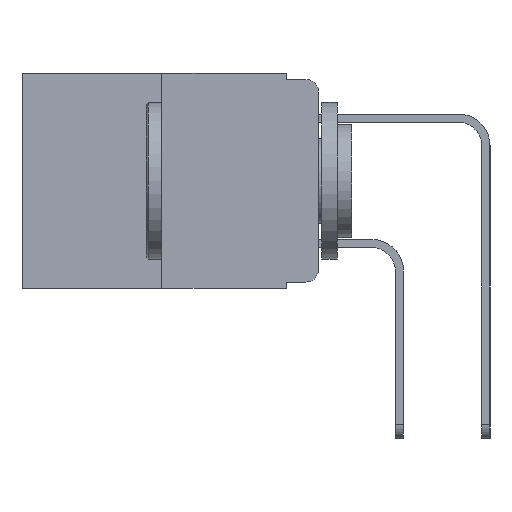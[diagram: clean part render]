
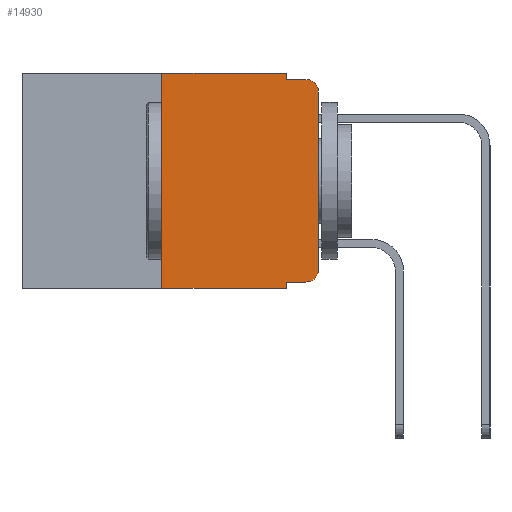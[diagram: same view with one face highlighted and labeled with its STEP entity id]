
A CAD part, left-side view. The second image highlights one B-rep face of the part: STEP entity #14930.
In plain terms, the highlighted planar face has unit normal (-1, 0, 0).
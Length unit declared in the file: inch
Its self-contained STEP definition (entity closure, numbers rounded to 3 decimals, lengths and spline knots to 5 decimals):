
#291 = DIRECTION ( 'NONE',  ( 0., 0., -1. ) ) ;
#442 = VERTEX_POINT ( 'NONE', #15512 ) ;
#761 = ORIENTED_EDGE ( 'NONE', *, *, #16289, .T. ) ;
#1004 = VECTOR ( 'NONE', #14730, 39.37008 ) ;
#1028 = ORIENTED_EDGE ( 'NONE', *, *, #16645, .F. ) ;
#1075 = VERTEX_POINT ( 'NONE', #9823 ) ;
#1347 = CARTESIAN_POINT ( 'NONE',  ( 0., 0.051, -0.01 ) ) ;
#1717 = FACE_OUTER_BOUND ( 'NONE', #5177, .T. ) ;
#1887 = LINE ( 'NONE', #19384, #17419 ) ;
#1895 = VERTEX_POINT ( 'NONE', #10454 ) ;
#1928 = VERTEX_POINT ( 'NONE', #13494 ) ;
#2020 = ORIENTED_EDGE ( 'NONE', *, *, #15933, .T. ) ;
#2046 = DIRECTION ( 'NONE',  ( 1., 0., 0. ) ) ;
#2171 = AXIS2_PLACEMENT_3D ( 'NONE', #11753, #2614, #13213 ) ;
#2304 = ORIENTED_EDGE ( 'NONE', *, *, #16283, .F. ) ;
#2614 = DIRECTION ( 'NONE',  ( -1., 0., 0. ) ) ;
#2619 = ORIENTED_EDGE ( 'NONE', *, *, #8684, .F. ) ;
#2909 = EDGE_CURVE ( 'NONE', #11151, #13283, #9089, .T. ) ;
#3618 = VECTOR ( 'NONE', #8699, 39.37008 ) ;
#3815 = DIRECTION ( 'NONE',  ( -1., 0., 0. ) ) ;
#3822 = CIRCLE ( 'NONE', #2171, 0.02 ) ;
#3830 = ORIENTED_EDGE ( 'NONE', *, *, #4227, .F. ) ;
#4227 = EDGE_CURVE ( 'NONE', #1895, #9646, #1887, .T. ) ;
#4546 = DIRECTION ( 'NONE',  ( 0., 0., 1. ) ) ;
#4596 = EDGE_CURVE ( 'NONE', #1075, #9885, #11877, .T. ) ;
#4952 = DIRECTION ( 'NONE',  ( 0., -1., 0. ) ) ;
#5177 = EDGE_LOOP ( 'NONE', ( #8118, #2020, #2304, #1028, #3830, #2619, #761, #13155, #13760, #7989 ) ) ;
#5407 = CARTESIAN_POINT ( 'NONE',  ( 0., 0.051, -0.343 ) ) ;
#5734 = CARTESIAN_POINT ( 'NONE',  ( 0., 0.051, -0.333 ) ) ;
#7221 = LINE ( 'NONE', #17619, #3618 ) ;
#7349 = CARTESIAN_POINT ( 'NONE',  ( 0., 0.02, -0.01 ) ) ;
#7453 = VERTEX_POINT ( 'NONE', #1347 ) ;
#7605 = DIRECTION ( 'NONE',  ( 0., -1., 0. ) ) ;
#7761 = LINE ( 'NONE', #15059, #15226 ) ;
#7989 = ORIENTED_EDGE ( 'NONE', *, *, #2909, .T. ) ;
#8118 = ORIENTED_EDGE ( 'NONE', *, *, #18871, .T. ) ;
#8357 = VECTOR ( 'NONE', #9488, 39.37008 ) ;
#8454 = CARTESIAN_POINT ( 'NONE',  ( 0., 0.051, 0. ) ) ;
#8684 = EDGE_CURVE ( 'NONE', #1928, #1895, #7761, .T. ) ;
#8699 = DIRECTION ( 'NONE',  ( 0., 0., 1. ) ) ;
#9057 = EDGE_CURVE ( 'NONE', #1075, #11151, #9170, .T. ) ;
#9089 = CIRCLE ( 'NONE', #19053, 0.02 ) ;
#9170 = LINE ( 'NONE', #5734, #1004 ) ;
#9416 = CARTESIAN_POINT ( 'NONE',  ( 0., 0.051, 0. ) ) ;
#9488 = DIRECTION ( 'NONE',  ( 0., -1., 0. ) ) ;
#9553 = CARTESIAN_POINT ( 'NONE',  ( 0., 0.473, -0.343 ) ) ;
#9646 = VERTEX_POINT ( 'NONE', #9416 ) ;
#9823 = CARTESIAN_POINT ( 'NONE',  ( 0., 0.051, -0.333 ) ) ;
#9885 = VERTEX_POINT ( 'NONE', #5407 ) ;
#10234 = VECTOR ( 'NONE', #291, 39.37008 ) ;
#10454 = CARTESIAN_POINT ( 'NONE',  ( 0., 0.25, 0. ) ) ;
#11019 = CARTESIAN_POINT ( 'NONE',  ( 0., 0.051, -0.01 ) ) ;
#11046 = CARTESIAN_POINT ( 'NONE',  ( 0., 0.051, 0. ) ) ;
#11079 = VERTEX_POINT ( 'NONE', #7349 ) ;
#11151 = VERTEX_POINT ( 'NONE', #19335 ) ;
#11193 = CARTESIAN_POINT ( 'NONE',  ( 0., 0.473, 0. ) ) ;
#11753 = CARTESIAN_POINT ( 'NONE',  ( 0., 0.02, -0.03 ) ) ;
#11877 = LINE ( 'NONE', #8454, #19201 ) ;
#12372 = LINE ( 'NONE', #11019, #8357 ) ;
#12682 = DIRECTION ( 'NONE',  ( 0., 0., -1. ) ) ;
#12841 = AXIS2_PLACEMENT_3D ( 'NONE', #11193, #2046, #12682 ) ;
#12901 = CARTESIAN_POINT ( 'NONE',  ( 0., 0.02, -0.313 ) ) ;
#13155 = ORIENTED_EDGE ( 'NONE', *, *, #4596, .F. ) ;
#13213 = DIRECTION ( 'NONE',  ( 0., 0., -1. ) ) ;
#13283 = VERTEX_POINT ( 'NONE', #17610 ) ;
#13494 = CARTESIAN_POINT ( 'NONE',  ( 0., 0.25, -0.343 ) ) ;
#13760 = ORIENTED_EDGE ( 'NONE', *, *, #9057, .T. ) ;
#14372 = DIRECTION ( 'NONE',  ( 0., 0., -1. ) ) ;
#14642 = LINE ( 'NONE', #11046, #10234 ) ;
#14730 = DIRECTION ( 'NONE',  ( 0., -1., 0. ) ) ;
#14930 = ADVANCED_FACE ( 'NONE', ( #1717 ), #18511, .F. ) ;
#15059 = CARTESIAN_POINT ( 'NONE',  ( 0., 0.25, 0. ) ) ;
#15226 = VECTOR ( 'NONE', #4546, 39.37008 ) ;
#15512 = CARTESIAN_POINT ( 'NONE',  ( 0., 0., -0.03 ) ) ;
#15933 = EDGE_CURVE ( 'NONE', #442, #11079, #3822, .T. ) ;
#16262 = VECTOR ( 'NONE', #4952, 39.37008 ) ;
#16283 = EDGE_CURVE ( 'NONE', #7453, #11079, #12372, .T. ) ;
#16289 = EDGE_CURVE ( 'NONE', #1928, #9885, #16723, .T. ) ;
#16645 = EDGE_CURVE ( 'NONE', #9646, #7453, #14642, .T. ) ;
#16723 = LINE ( 'NONE', #9553, #16262 ) ;
#17419 = VECTOR ( 'NONE', #7605, 39.37008 ) ;
#17610 = CARTESIAN_POINT ( 'NONE',  ( 0., 0., -0.313 ) ) ;
#17619 = CARTESIAN_POINT ( 'NONE',  ( 0., 0., 0. ) ) ;
#18511 = PLANE ( 'NONE',  #12841 ) ;
#18819 = DIRECTION ( 'NONE',  ( 0., 0., -1. ) ) ;
#18871 = EDGE_CURVE ( 'NONE', #13283, #442, #7221, .T. ) ;
#19053 = AXIS2_PLACEMENT_3D ( 'NONE', #12901, #3815, #14372 ) ;
#19201 = VECTOR ( 'NONE', #18819, 39.37008 ) ;
#19335 = CARTESIAN_POINT ( 'NONE',  ( 0., 0.02, -0.333 ) ) ;
#19384 = CARTESIAN_POINT ( 'NONE',  ( 0., 0.473, 0. ) ) ;
